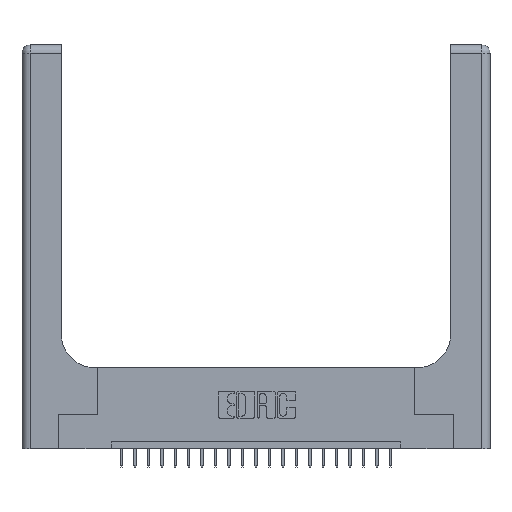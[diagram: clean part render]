
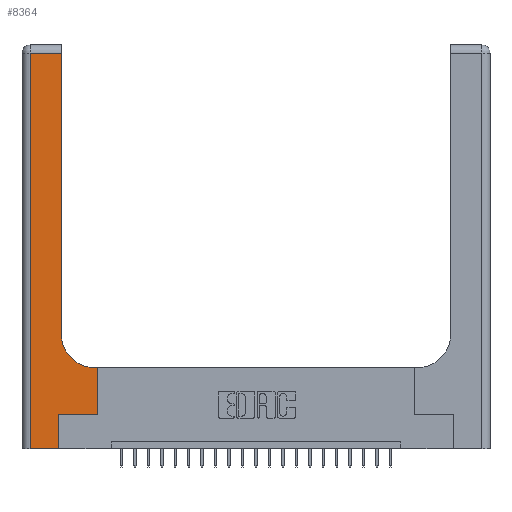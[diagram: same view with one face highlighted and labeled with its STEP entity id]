
A CAD part, top view. The second image highlights one B-rep face of the part: STEP entity #8364.
In plain terms, the highlighted planar face has unit normal (0, 0, 1).
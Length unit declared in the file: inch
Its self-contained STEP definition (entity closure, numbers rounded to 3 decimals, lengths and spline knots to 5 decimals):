
#581 = CARTESIAN_POINT ( 'NONE',  ( 0.5415, 0.85, 0.37 ) ) ;
#942 = ORIENTED_EDGE ( 'NONE', *, *, #1953, .T. ) ;
#1024 = VERTEX_POINT ( 'NONE', #15427 ) ;
#1035 = CARTESIAN_POINT ( 'NONE',  ( 0.2915, 0.85, 0.37 ) ) ;
#1557 = EDGE_CURVE ( 'NONE', #6568, #18835, #22719, .T. ) ;
#1781 = EDGE_CURVE ( 'NONE', #13255, #6568, #12700, .T. ) ;
#1953 = EDGE_CURVE ( 'NONE', #9666, #9347, #6438, .T. ) ;
#2084 = EDGE_CURVE ( 'NONE', #5918, #9666, #20369, .T. ) ;
#2118 = VECTOR ( 'NONE', #16446, 39.37008 ) ;
#2201 = ORIENTED_EDGE ( 'NONE', *, *, #1781, .T. ) ;
#2697 = PLANE ( 'NONE',  #21600 ) ;
#2769 = CARTESIAN_POINT ( 'NONE',  ( 0.2915, 2.94, 0.37 ) ) ;
#2873 = VECTOR ( 'NONE', #3057, 39.37008 ) ;
#3057 = DIRECTION ( 'NONE',  ( 0., 1., 0. ) ) ;
#3278 = EDGE_CURVE ( 'NONE', #9347, #19905, #12203, .T. ) ;
#4207 = AXIS2_PLACEMENT_3D ( 'NONE', #581, #15138, #9586 ) ;
#4294 = DIRECTION ( 'NONE',  ( 0., 1., 0. ) ) ;
#4325 = EDGE_CURVE ( 'NONE', #12247, #1024, #9105, .T. ) ;
#4352 = CARTESIAN_POINT ( 'NONE',  ( 0.5585, 0.6, 0.37 ) ) ;
#4514 = DIRECTION ( 'NONE',  ( 1., 0., 0. ) ) ;
#4869 = CARTESIAN_POINT ( 'NONE',  ( 0.269, 0.25, 0.37 ) ) ;
#5528 = CARTESIAN_POINT ( 'NONE',  ( 0.2915, 0.6, 0.37 ) ) ;
#5895 = ORIENTED_EDGE ( 'NONE', *, *, #1557, .T. ) ;
#5918 = VERTEX_POINT ( 'NONE', #16704 ) ;
#5993 = VECTOR ( 'NONE', #4514, 39.37008 ) ;
#6114 = CARTESIAN_POINT ( 'NONE',  ( 0., 2.94, 0.37 ) ) ;
#6438 = LINE ( 'NONE', #19310, #2873 ) ;
#6568 = VERTEX_POINT ( 'NONE', #2769 ) ;
#6732 = DIRECTION ( 'NONE',  ( 0., -1., 0. ) ) ;
#6918 = DIRECTION ( 'NONE',  ( 1., 0., 0. ) ) ;
#7096 = CARTESIAN_POINT ( 'NONE',  ( 0.269, 0.25, 0.37 ) ) ;
#7996 = CARTESIAN_POINT ( 'NONE',  ( 0.5585, 0.25, 0.37 ) ) ;
#8364 = ADVANCED_FACE ( 'NONE', ( #10135 ), #2697, .F. ) ;
#9028 = VECTOR ( 'NONE', #6732, 39.37008 ) ;
#9105 = LINE ( 'NONE', #5528, #2118 ) ;
#9212 = CARTESIAN_POINT ( 'NONE',  ( 0.06, 2.94, 0.37 ) ) ;
#9347 = VERTEX_POINT ( 'NONE', #7096 ) ;
#9512 = ORIENTED_EDGE ( 'NONE', *, *, #2084, .T. ) ;
#9586 = DIRECTION ( 'NONE',  ( 1., 0., 0. ) ) ;
#9666 = VERTEX_POINT ( 'NONE', #17442 ) ;
#9931 = CARTESIAN_POINT ( 'NONE',  ( 0.5585, 0.25, 0.37 ) ) ;
#10135 = FACE_OUTER_BOUND ( 'NONE', #12673, .T. ) ;
#10364 = DIRECTION ( 'NONE',  ( -1., 0., 0. ) ) ;
#11510 = LINE ( 'NONE', #9931, #20727 ) ;
#12203 = LINE ( 'NONE', #4869, #5993 ) ;
#12247 = VERTEX_POINT ( 'NONE', #4352 ) ;
#12349 = ORIENTED_EDGE ( 'NONE', *, *, #19016, .T. ) ;
#12673 = EDGE_LOOP ( 'NONE', ( #2201, #5895, #18982, #9512, #942, #14513, #12349, #18567, #15794 ) ) ;
#12700 = LINE ( 'NONE', #20396, #14110 ) ;
#12834 = EDGE_CURVE ( 'NONE', #18835, #5918, #14053, .T. ) ;
#13255 = VERTEX_POINT ( 'NONE', #1035 ) ;
#13566 = DIRECTION ( 'NONE',  ( -1., 0., 0. ) ) ;
#13826 = CARTESIAN_POINT ( 'NONE',  ( 0.06, 3., 0.37 ) ) ;
#14053 = LINE ( 'NONE', #13826, #9028 ) ;
#14110 = VECTOR ( 'NONE', #20034, 39.37008 ) ;
#14513 = ORIENTED_EDGE ( 'NONE', *, *, #3278, .T. ) ;
#14693 = CIRCLE ( 'NONE', #4207, 0.25 ) ;
#15138 = DIRECTION ( 'NONE',  ( 0., 0., -1. ) ) ;
#15427 = CARTESIAN_POINT ( 'NONE',  ( 0.5415, 0.6, 0.37 ) ) ;
#15794 = ORIENTED_EDGE ( 'NONE', *, *, #20246, .T. ) ;
#16446 = DIRECTION ( 'NONE',  ( -1., 0., 0. ) ) ;
#16704 = CARTESIAN_POINT ( 'NONE',  ( 0.06, 0., 0.37 ) ) ;
#17442 = CARTESIAN_POINT ( 'NONE',  ( 0.269, 0., 0.37 ) ) ;
#17946 = VECTOR ( 'NONE', #6918, 39.37008 ) ;
#18567 = ORIENTED_EDGE ( 'NONE', *, *, #4325, .T. ) ;
#18835 = VERTEX_POINT ( 'NONE', #9212 ) ;
#18982 = ORIENTED_EDGE ( 'NONE', *, *, #12834, .T. ) ;
#19016 = EDGE_CURVE ( 'NONE', #19905, #12247, #11510, .T. ) ;
#19062 = CARTESIAN_POINT ( 'NONE',  ( 0., 3., 0.37 ) ) ;
#19310 = CARTESIAN_POINT ( 'NONE',  ( 0.269, 0., 0.37 ) ) ;
#19413 = DIRECTION ( 'NONE',  ( 0., 0., -1. ) ) ;
#19905 = VERTEX_POINT ( 'NONE', #7996 ) ;
#20034 = DIRECTION ( 'NONE',  ( 0., 1., 0. ) ) ;
#20246 = EDGE_CURVE ( 'NONE', #1024, #13255, #14693, .T. ) ;
#20369 = LINE ( 'NONE', #21839, #17946 ) ;
#20396 = CARTESIAN_POINT ( 'NONE',  ( 0.2915, 3., 0.37 ) ) ;
#20727 = VECTOR ( 'NONE', #4294, 39.37008 ) ;
#21600 = AXIS2_PLACEMENT_3D ( 'NONE', #19062, #19413, #10364 ) ;
#21808 = VECTOR ( 'NONE', #13566, 39.37008 ) ;
#21839 = CARTESIAN_POINT ( 'NONE',  ( 0., 0., 0.37 ) ) ;
#22719 = LINE ( 'NONE', #6114, #21808 ) ;
